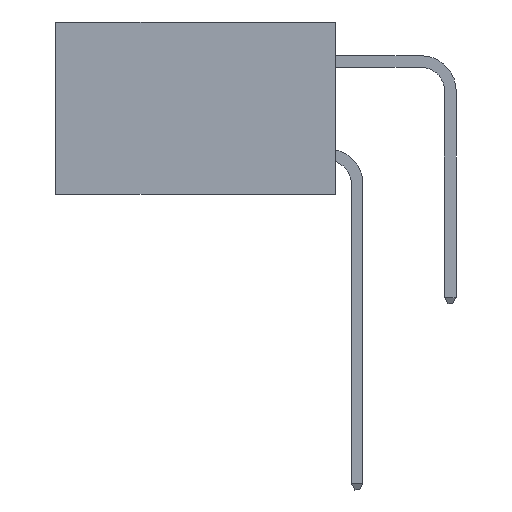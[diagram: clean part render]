
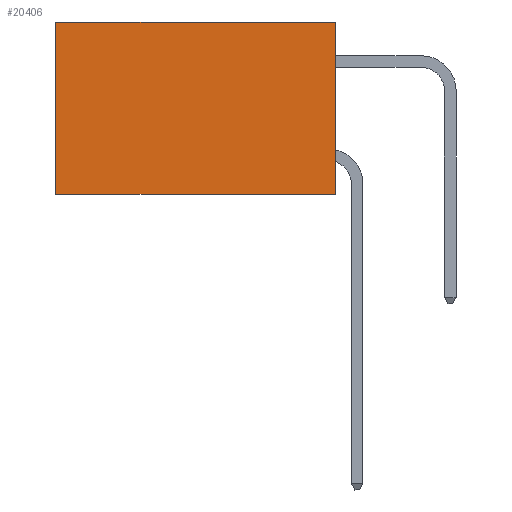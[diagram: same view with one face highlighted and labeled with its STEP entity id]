
A CAD part, left-side view. The second image highlights one B-rep face of the part: STEP entity #20406.
In plain terms, the highlighted planar face has unit normal (-1, 0, 0).
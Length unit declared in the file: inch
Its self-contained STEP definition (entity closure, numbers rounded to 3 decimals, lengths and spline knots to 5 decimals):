
#897 = EDGE_CURVE ( 'NONE', #1197, #13815, #5314, .T. ) ;
#1197 = VERTEX_POINT ( 'NONE', #1327 ) ;
#1284 = DIRECTION ( 'NONE',  ( 0., 1., 0. ) ) ;
#1327 = CARTESIAN_POINT ( 'NONE',  ( 0.2875, 0., -0.37 ) ) ;
#1455 = LINE ( 'NONE', #18435, #13948 ) ;
#4110 = VECTOR ( 'NONE', #7196, 39.37008 ) ;
#4169 = DIRECTION ( 'NONE',  ( 1., 0., 0. ) ) ;
#4242 = VECTOR ( 'NONE', #18505, 39.37008 ) ;
#4369 = VERTEX_POINT ( 'NONE', #12595 ) ;
#5138 = FACE_OUTER_BOUND ( 'NONE', #12147, .T. ) ;
#5296 = CARTESIAN_POINT ( 'NONE',  ( 0.2875, 0., -0.37 ) ) ;
#5314 = LINE ( 'NONE', #5296, #4110 ) ;
#6891 = LINE ( 'NONE', #16972, #16829 ) ;
#7196 = DIRECTION ( 'NONE',  ( 0., 1., 0. ) ) ;
#8563 = ORIENTED_EDGE ( 'NONE', *, *, #19016, .T. ) ;
#8698 = AXIS2_PLACEMENT_3D ( 'NONE', #13703, #4169, #19746 ) ;
#9609 = ORIENTED_EDGE ( 'NONE', *, *, #14788, .T. ) ;
#10855 = CARTESIAN_POINT ( 'NONE',  ( 0.2875, 0., 0. ) ) ;
#12147 = EDGE_LOOP ( 'NONE', ( #9609, #13236, #15103, #8563 ) ) ;
#12204 = CARTESIAN_POINT ( 'NONE',  ( 0.2875, 0.6, 0. ) ) ;
#12595 = CARTESIAN_POINT ( 'NONE',  ( 0.2875, 0.6, 0. ) ) ;
#12679 = CARTESIAN_POINT ( 'NONE',  ( 0.2875, 0.6, -0.37 ) ) ;
#13236 = ORIENTED_EDGE ( 'NONE', *, *, #897, .F. ) ;
#13703 = CARTESIAN_POINT ( 'NONE',  ( 0.2875, 0., 0. ) ) ;
#13815 = VERTEX_POINT ( 'NONE', #12679 ) ;
#13878 = DIRECTION ( 'NONE',  ( 0., 0., -1. ) ) ;
#13948 = VECTOR ( 'NONE', #1284, 39.37008 ) ;
#14788 = EDGE_CURVE ( 'NONE', #4369, #13815, #18689, .T. ) ;
#14799 = EDGE_CURVE ( 'NONE', #17762, #1197, #6891, .T. ) ;
#15103 = ORIENTED_EDGE ( 'NONE', *, *, #14799, .F. ) ;
#15266 = PLANE ( 'NONE',  #8698 ) ;
#16829 = VECTOR ( 'NONE', #13878, 39.37008 ) ;
#16972 = CARTESIAN_POINT ( 'NONE',  ( 0.2875, 0., 0. ) ) ;
#17762 = VERTEX_POINT ( 'NONE', #10855 ) ;
#18435 = CARTESIAN_POINT ( 'NONE',  ( 0.2875, 0., 0. ) ) ;
#18505 = DIRECTION ( 'NONE',  ( 0., 0., -1. ) ) ;
#18689 = LINE ( 'NONE', #12204, #4242 ) ;
#19016 = EDGE_CURVE ( 'NONE', #17762, #4369, #1455, .T. ) ;
#19746 = DIRECTION ( 'NONE',  ( 0., 0., -1. ) ) ;
#20406 = ADVANCED_FACE ( 'NONE', ( #5138 ), #15266, .F. ) ;
